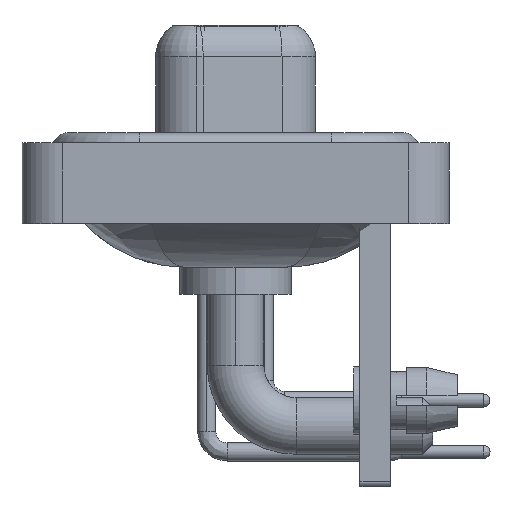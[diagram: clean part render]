
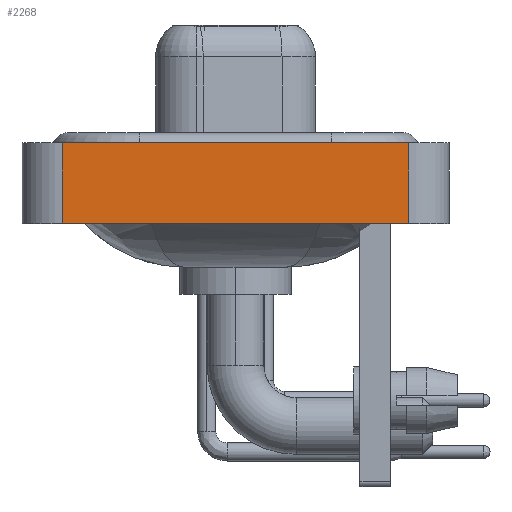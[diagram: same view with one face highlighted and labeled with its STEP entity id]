
A CAD part, left-side view. The second image highlights one B-rep face of the part: STEP entity #2268.
In plain terms, the highlighted planar face has unit normal (-1, 0, 0).
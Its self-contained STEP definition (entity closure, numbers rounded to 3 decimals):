
#971 = CARTESIAN_POINT ( 'NONE',  ( -7.35, -8.55, -3.6 ) ) ;
#1159 = ORIENTED_EDGE ( 'NONE', *, *, #6245, .F. ) ;
#2268 = ADVANCED_FACE ( 'NONE', ( #10501 ), #16150, .T. ) ;
#2484 = LINE ( 'NONE', #18979, #6687 ) ;
#4028 = ORIENTED_EDGE ( 'NONE', *, *, #16409, .F. ) ;
#4167 = DIRECTION ( 'NONE',  ( 0., 0., 1. ) ) ;
#4482 = EDGE_CURVE ( 'NONE', #18989, #21415, #20548, .T. ) ;
#4785 = LINE ( 'NONE', #971, #13867 ) ;
#5291 = CARTESIAN_POINT ( 'NONE',  ( -7.35, 8.55, -3.6 ) ) ;
#5559 = CARTESIAN_POINT ( 'NONE',  ( -7.35, -8.55, -3.6 ) ) ;
#5722 = EDGE_CURVE ( 'NONE', #14768, #18989, #4785, .T. ) ;
#6245 = EDGE_CURVE ( 'NONE', #14768, #17443, #2484, .T. ) ;
#6687 = VECTOR ( 'NONE', #8419, 1000. ) ;
#6908 = DIRECTION ( 'NONE',  ( -1., 0., 0. ) ) ;
#7278 = ORIENTED_EDGE ( 'NONE', *, *, #5722, .T. ) ;
#7353 = CARTESIAN_POINT ( 'NONE',  ( -7.35, -8.55, -3.6 ) ) ;
#8419 = DIRECTION ( 'NONE',  ( 0., 0., 1. ) ) ;
#9056 = AXIS2_PLACEMENT_3D ( 'NONE', #7353, #6908, #10841 ) ;
#9749 = CARTESIAN_POINT ( 'NONE',  ( -7.35, -8.55, -3.6 ) ) ;
#10457 = CARTESIAN_POINT ( 'NONE',  ( -7.35, 8.55, 0.4 ) ) ;
#10501 = FACE_OUTER_BOUND ( 'NONE', #21406, .T. ) ;
#10841 = DIRECTION ( 'NONE',  ( 0., 0., 1. ) ) ;
#12559 = DIRECTION ( 'NONE',  ( 0., -1., 0. ) ) ;
#13792 = VECTOR ( 'NONE', #4167, 1000. ) ;
#13867 = VECTOR ( 'NONE', #13946, 1000. ) ;
#13946 = DIRECTION ( 'NONE',  ( 0., -1., 0. ) ) ;
#14768 = VERTEX_POINT ( 'NONE', #5291 ) ;
#15734 = CARTESIAN_POINT ( 'NONE',  ( -7.35, -8.55, 0.4 ) ) ;
#16150 = PLANE ( 'NONE',  #9056 ) ;
#16409 = EDGE_CURVE ( 'NONE', #17443, #21415, #23272, .T. ) ;
#17443 = VERTEX_POINT ( 'NONE', #10457 ) ;
#18979 = CARTESIAN_POINT ( 'NONE',  ( -7.35, 8.55, -3.6 ) ) ;
#18989 = VERTEX_POINT ( 'NONE', #5559 ) ;
#20548 = LINE ( 'NONE', #9749, #13792 ) ;
#21092 = CARTESIAN_POINT ( 'NONE',  ( -7.35, -8.55, 0.4 ) ) ;
#21394 = VECTOR ( 'NONE', #12559, 1000. ) ;
#21406 = EDGE_LOOP ( 'NONE', ( #23116, #4028, #1159, #7278 ) ) ;
#21415 = VERTEX_POINT ( 'NONE', #21092 ) ;
#23116 = ORIENTED_EDGE ( 'NONE', *, *, #4482, .T. ) ;
#23272 = LINE ( 'NONE', #15734, #21394 ) ;
